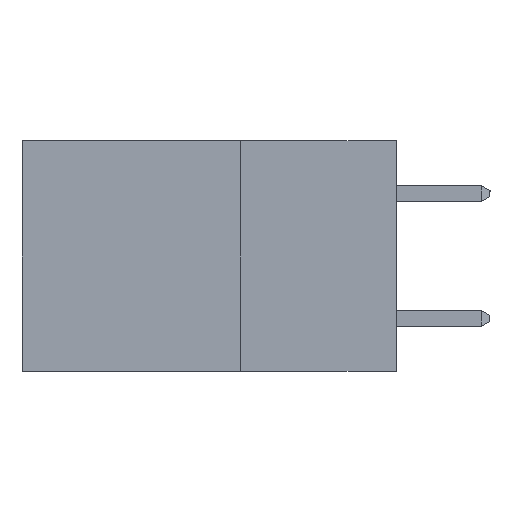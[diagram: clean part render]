
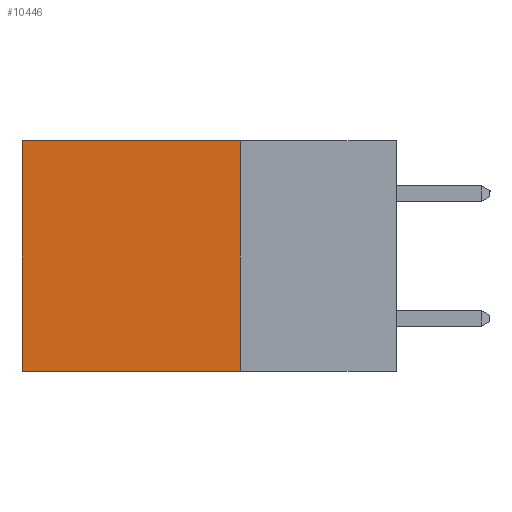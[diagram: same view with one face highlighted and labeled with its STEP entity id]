
A CAD part, left-side view. The second image highlights one B-rep face of the part: STEP entity #10446.
In plain terms, the highlighted planar face has unit normal (-1, 0, 0).
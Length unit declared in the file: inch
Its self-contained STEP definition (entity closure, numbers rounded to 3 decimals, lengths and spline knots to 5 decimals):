
#438 = ORIENTED_EDGE ( 'NONE', *, *, #10568, .F. ) ;
#445 = EDGE_CURVE ( 'NONE', #854, #1268, #7762, .T. ) ;
#854 = VERTEX_POINT ( 'NONE', #9497 ) ;
#1061 = DIRECTION ( 'NONE',  ( 0., 0., -1. ) ) ;
#1068 = VECTOR ( 'NONE', #10146, 39.37008 ) ;
#1127 = LINE ( 'NONE', #8219, #1068 ) ;
#1268 = VERTEX_POINT ( 'NONE', #4031 ) ;
#1674 = DIRECTION ( 'NONE',  ( 0., 0., -1. ) ) ;
#1731 = VERTEX_POINT ( 'NONE', #9682 ) ;
#1993 = CARTESIAN_POINT ( 'NONE',  ( 0.2615, 0.25, -0.37 ) ) ;
#2390 = CARTESIAN_POINT ( 'NONE',  ( 0.2615, 0.6, -0.37 ) ) ;
#2775 = FACE_OUTER_BOUND ( 'NONE', #7410, .T. ) ;
#2850 = ORIENTED_EDGE ( 'NONE', *, *, #11242, .F. ) ;
#3671 = CARTESIAN_POINT ( 'NONE',  ( 0.2615, 0.25, -0.37 ) ) ;
#3819 = VERTEX_POINT ( 'NONE', #4106 ) ;
#4031 = CARTESIAN_POINT ( 'NONE',  ( 0.2615, 0.6, -0.37 ) ) ;
#4106 = CARTESIAN_POINT ( 'NONE',  ( 0.2615, 0.25, 0. ) ) ;
#4160 = EDGE_CURVE ( 'NONE', #3819, #854, #1127, .T. ) ;
#4615 = ORIENTED_EDGE ( 'NONE', *, *, #445, .T. ) ;
#5390 = DIRECTION ( 'NONE',  ( 1., 0., 0. ) ) ;
#6397 = DIRECTION ( 'NONE',  ( 0., 0., -1. ) ) ;
#7169 = ORIENTED_EDGE ( 'NONE', *, *, #4160, .T. ) ;
#7410 = EDGE_LOOP ( 'NONE', ( #4615, #438, #2850, #7169 ) ) ;
#7762 = LINE ( 'NONE', #2390, #8508 ) ;
#8198 = PLANE ( 'NONE',  #10145 ) ;
#8219 = CARTESIAN_POINT ( 'NONE',  ( 0.2615, 0.25, 0. ) ) ;
#8508 = VECTOR ( 'NONE', #1674, 39.37008 ) ;
#8851 = VECTOR ( 'NONE', #1061, 39.37008 ) ;
#9147 = LINE ( 'NONE', #3671, #8851 ) ;
#9360 = LINE ( 'NONE', #1993, #10693 ) ;
#9497 = CARTESIAN_POINT ( 'NONE',  ( 0.2615, 0.6, 0. ) ) ;
#9682 = CARTESIAN_POINT ( 'NONE',  ( 0.2615, 0.25, -0.37 ) ) ;
#9832 = CARTESIAN_POINT ( 'NONE',  ( 0.2615, 0.25, -0.37 ) ) ;
#10145 = AXIS2_PLACEMENT_3D ( 'NONE', #9832, #5390, #6397 ) ;
#10146 = DIRECTION ( 'NONE',  ( 0., 1., 0. ) ) ;
#10446 = ADVANCED_FACE ( 'NONE', ( #2775 ), #8198, .F. ) ;
#10568 = EDGE_CURVE ( 'NONE', #1731, #1268, #9360, .T. ) ;
#10693 = VECTOR ( 'NONE', #11050, 39.37008 ) ;
#11050 = DIRECTION ( 'NONE',  ( 0., 1., 0. ) ) ;
#11242 = EDGE_CURVE ( 'NONE', #3819, #1731, #9147, .T. ) ;
